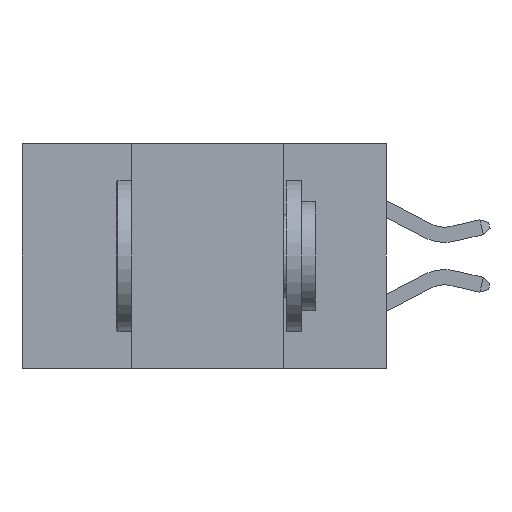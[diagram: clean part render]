
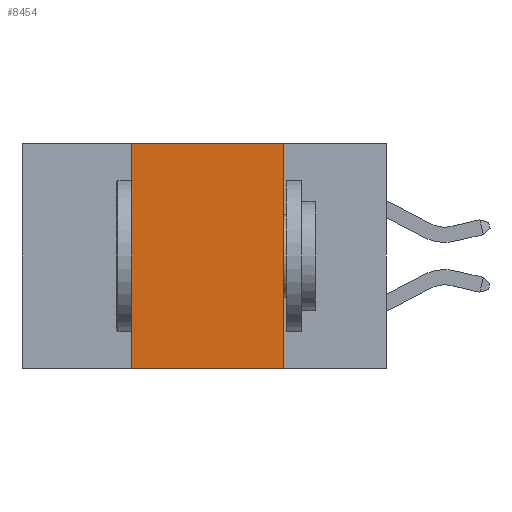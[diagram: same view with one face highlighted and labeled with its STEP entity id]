
A CAD part, left-side view. The second image highlights one B-rep face of the part: STEP entity #8454.
In plain terms, the highlighted planar face has unit normal (-1, 0, 0).
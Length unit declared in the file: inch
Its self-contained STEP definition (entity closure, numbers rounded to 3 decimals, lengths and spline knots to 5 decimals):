
#376 = DIRECTION ( 'NONE',  ( 0., -1., 0. ) ) ;
#850 = CARTESIAN_POINT ( 'NONE',  ( 0., 0.17, 0. ) ) ;
#1491 = DIRECTION ( 'NONE',  ( 0., 0., 1. ) ) ;
#2557 = AXIS2_PLACEMENT_3D ( 'NONE', #10049, #16010, #16485 ) ;
#2831 = LINE ( 'NONE', #17616, #14645 ) ;
#2849 = VECTOR ( 'NONE', #376, 39.37008 ) ;
#3782 = VECTOR ( 'NONE', #15601, 39.37008 ) ;
#3832 = CARTESIAN_POINT ( 'NONE',  ( 0., 0.17, -0.37 ) ) ;
#3926 = VERTEX_POINT ( 'NONE', #13807 ) ;
#4077 = PLANE ( 'NONE',  #2557 ) ;
#6055 = ORIENTED_EDGE ( 'NONE', *, *, #10118, .F. ) ;
#6583 = EDGE_CURVE ( 'NONE', #13732, #18391, #2831, .T. ) ;
#6995 = ORIENTED_EDGE ( 'NONE', *, *, #6583, .T. ) ;
#7023 = FACE_OUTER_BOUND ( 'NONE', #18528, .T. ) ;
#8454 = ADVANCED_FACE ( 'NONE', ( #7023 ), #4077, .F. ) ;
#8521 = CARTESIAN_POINT ( 'NONE',  ( 0., 0.42, -0.37 ) ) ;
#8581 = EDGE_CURVE ( 'NONE', #3926, #8718, #13641, .T. ) ;
#8718 = VERTEX_POINT ( 'NONE', #850 ) ;
#8813 = LINE ( 'NONE', #17932, #10701 ) ;
#9050 = CARTESIAN_POINT ( 'NONE',  ( 0., 0.6, 0. ) ) ;
#9641 = CARTESIAN_POINT ( 'NONE',  ( 0., 0.17, -0.37 ) ) ;
#10049 = CARTESIAN_POINT ( 'NONE',  ( 0., 0.6, 0. ) ) ;
#10118 = EDGE_CURVE ( 'NONE', #13732, #3926, #8813, .T. ) ;
#10163 = DIRECTION ( 'NONE',  ( 0., -1., 0. ) ) ;
#10701 = VECTOR ( 'NONE', #1491, 39.37008 ) ;
#11064 = ORIENTED_EDGE ( 'NONE', *, *, #8581, .F. ) ;
#13641 = LINE ( 'NONE', #9050, #2849 ) ;
#13732 = VERTEX_POINT ( 'NONE', #8521 ) ;
#13807 = CARTESIAN_POINT ( 'NONE',  ( 0., 0.42, 0. ) ) ;
#14645 = VECTOR ( 'NONE', #10163, 39.37008 ) ;
#14732 = ORIENTED_EDGE ( 'NONE', *, *, #19250, .F. ) ;
#15601 = DIRECTION ( 'NONE',  ( 0., 0., -1. ) ) ;
#16010 = DIRECTION ( 'NONE',  ( 1., 0., 0. ) ) ;
#16485 = DIRECTION ( 'NONE',  ( 0., 0., -1. ) ) ;
#17188 = LINE ( 'NONE', #9641, #3782 ) ;
#17616 = CARTESIAN_POINT ( 'NONE',  ( 0., 0.6, -0.37 ) ) ;
#17932 = CARTESIAN_POINT ( 'NONE',  ( 0., 0.42, -0.37 ) ) ;
#18391 = VERTEX_POINT ( 'NONE', #3832 ) ;
#18528 = EDGE_LOOP ( 'NONE', ( #14732, #11064, #6055, #6995 ) ) ;
#19250 = EDGE_CURVE ( 'NONE', #8718, #18391, #17188, .T. ) ;
